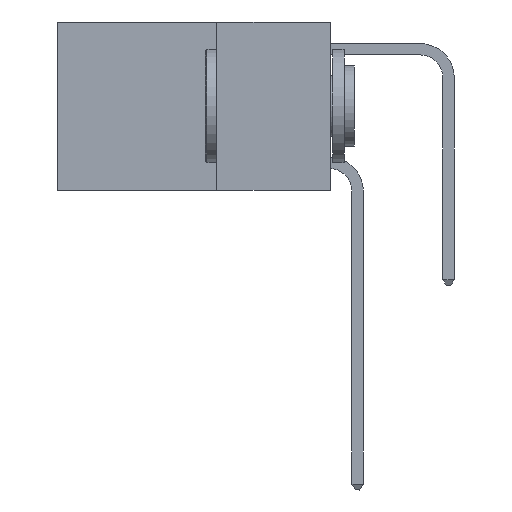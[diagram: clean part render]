
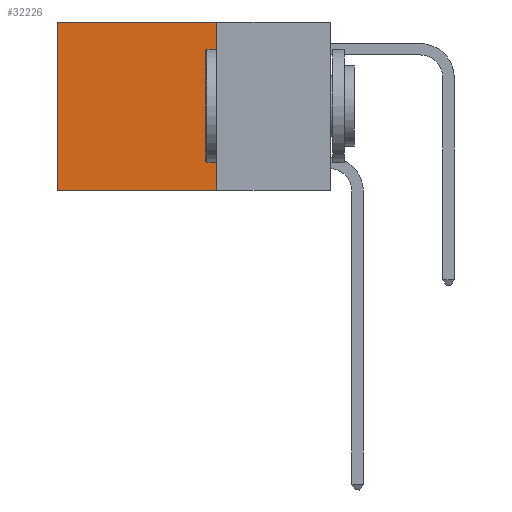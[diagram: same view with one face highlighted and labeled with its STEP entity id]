
A CAD part, left-side view. The second image highlights one B-rep face of the part: STEP entity #32226.
In plain terms, the highlighted planar face has unit normal (-1, 0, 0).
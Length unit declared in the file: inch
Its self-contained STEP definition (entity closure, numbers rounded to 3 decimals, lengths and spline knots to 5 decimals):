
#26 = CARTESIAN_POINT ( 'NONE',  ( 0.2625, 0.25, 0. ) ) ;
#1394 = DIRECTION ( 'NONE',  ( 0., 0., -1. ) ) ;
#1607 = FACE_OUTER_BOUND ( 'NONE', #23440, .T. ) ;
#1852 = ORIENTED_EDGE ( 'NONE', *, *, #3587, .T. ) ;
#3587 = EDGE_CURVE ( 'NONE', #6474, #17224, #7518, .T. ) ;
#6474 = VERTEX_POINT ( 'NONE', #24383 ) ;
#6578 = ORIENTED_EDGE ( 'NONE', *, *, #14884, .T. ) ;
#7518 = LINE ( 'NONE', #13108, #24017 ) ;
#8316 = VECTOR ( 'NONE', #1394, 39.37008 ) ;
#8496 = PLANE ( 'NONE',  #14754 ) ;
#9536 = CARTESIAN_POINT ( 'NONE',  ( 0.2625, 0.6, 0. ) ) ;
#9784 = DIRECTION ( 'NONE',  ( 0., 0., -1. ) ) ;
#10748 = VECTOR ( 'NONE', #14386, 39.37008 ) ;
#13108 = CARTESIAN_POINT ( 'NONE',  ( 0.2625, 0.25, 0. ) ) ;
#13529 = DIRECTION ( 'NONE',  ( 0., 0., -1. ) ) ;
#14386 = DIRECTION ( 'NONE',  ( 0., 1., 0. ) ) ;
#14754 = AXIS2_PLACEMENT_3D ( 'NONE', #23954, #28912, #13529 ) ;
#14884 = EDGE_CURVE ( 'NONE', #17224, #21424, #25640, .T. ) ;
#16847 = CARTESIAN_POINT ( 'NONE',  ( 0.2625, 0.6, 0. ) ) ;
#17224 = VERTEX_POINT ( 'NONE', #9536 ) ;
#18183 = LINE ( 'NONE', #19210, #10748 ) ;
#19210 = CARTESIAN_POINT ( 'NONE',  ( 0.2625, 0.25, -0.37 ) ) ;
#21263 = ORIENTED_EDGE ( 'NONE', *, *, #23648, .F. ) ;
#21424 = VERTEX_POINT ( 'NONE', #26138 ) ;
#21660 = EDGE_CURVE ( 'NONE', #23836, #21424, #18183, .T. ) ;
#23211 = VECTOR ( 'NONE', #9784, 39.37008 ) ;
#23440 = EDGE_LOOP ( 'NONE', ( #6578, #32336, #21263, #1852 ) ) ;
#23648 = EDGE_CURVE ( 'NONE', #6474, #23836, #27572, .T. ) ;
#23836 = VERTEX_POINT ( 'NONE', #28056 ) ;
#23954 = CARTESIAN_POINT ( 'NONE',  ( 0.2625, 0.25, 0. ) ) ;
#24017 = VECTOR ( 'NONE', #25660, 39.37008 ) ;
#24383 = CARTESIAN_POINT ( 'NONE',  ( 0.2625, 0.25, 0. ) ) ;
#25640 = LINE ( 'NONE', #16847, #8316 ) ;
#25660 = DIRECTION ( 'NONE',  ( 0., 1., 0. ) ) ;
#26138 = CARTESIAN_POINT ( 'NONE',  ( 0.2625, 0.6, -0.37 ) ) ;
#27572 = LINE ( 'NONE', #26, #23211 ) ;
#28056 = CARTESIAN_POINT ( 'NONE',  ( 0.2625, 0.25, -0.37 ) ) ;
#28912 = DIRECTION ( 'NONE',  ( 1., 0., 0. ) ) ;
#32226 = ADVANCED_FACE ( 'NONE', ( #1607 ), #8496, .F. ) ;
#32336 = ORIENTED_EDGE ( 'NONE', *, *, #21660, .F. ) ;
